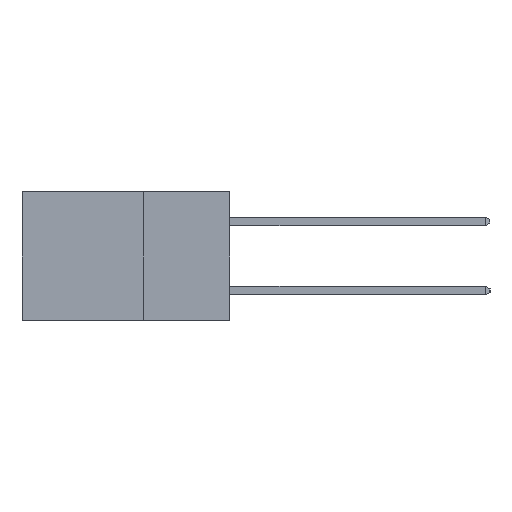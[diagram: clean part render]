
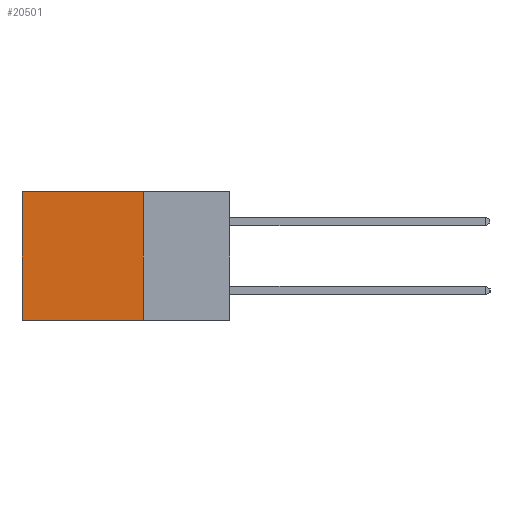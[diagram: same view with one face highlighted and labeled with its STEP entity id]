
A CAD part, left-side view. The second image highlights one B-rep face of the part: STEP entity #20501.
In plain terms, the highlighted planar face has unit normal (-1, 0, 0).
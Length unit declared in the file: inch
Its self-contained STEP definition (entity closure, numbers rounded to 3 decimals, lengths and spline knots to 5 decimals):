
#263 = CARTESIAN_POINT ( 'NONE',  ( 0.2615, 0.25, -0.37 ) ) ;
#494 = EDGE_CURVE ( 'NONE', #7256, #14960, #4353, .T. ) ;
#1299 = VERTEX_POINT ( 'NONE', #11297 ) ;
#1305 = CARTESIAN_POINT ( 'NONE',  ( 0.2615, 0.25, -0.37 ) ) ;
#1597 = FACE_OUTER_BOUND ( 'NONE', #7413, .T. ) ;
#2206 = LINE ( 'NONE', #10711, #11659 ) ;
#2581 = CARTESIAN_POINT ( 'NONE',  ( 0.2615, 0.25, -0.37 ) ) ;
#4353 = LINE ( 'NONE', #13115, #24732 ) ;
#5641 = EDGE_CURVE ( 'NONE', #7256, #10515, #22457, .T. ) ;
#6555 = DIRECTION ( 'NONE',  ( 1., 0., 0. ) ) ;
#7256 = VERTEX_POINT ( 'NONE', #17241 ) ;
#7413 = EDGE_LOOP ( 'NONE', ( #18184, #19885, #15107, #17958 ) ) ;
#7924 = VECTOR ( 'NONE', #14246, 39.37008 ) ;
#10231 = VECTOR ( 'NONE', #24812, 39.37008 ) ;
#10515 = VERTEX_POINT ( 'NONE', #10915 ) ;
#10711 = CARTESIAN_POINT ( 'NONE',  ( 0.2615, 0.6, -0.37 ) ) ;
#10915 = CARTESIAN_POINT ( 'NONE',  ( 0.2615, 0.25, -0.37 ) ) ;
#11297 = CARTESIAN_POINT ( 'NONE',  ( 0.2615, 0.6, -0.37 ) ) ;
#11659 = VECTOR ( 'NONE', #24363, 39.37008 ) ;
#13115 = CARTESIAN_POINT ( 'NONE',  ( 0.2615, 0.25, 0. ) ) ;
#14110 = EDGE_CURVE ( 'NONE', #14960, #1299, #2206, .T. ) ;
#14246 = DIRECTION ( 'NONE',  ( 0., 0., -1. ) ) ;
#14960 = VERTEX_POINT ( 'NONE', #22889 ) ;
#15107 = ORIENTED_EDGE ( 'NONE', *, *, #5641, .F. ) ;
#15469 = AXIS2_PLACEMENT_3D ( 'NONE', #2581, #6555, #20444 ) ;
#16150 = EDGE_CURVE ( 'NONE', #10515, #1299, #18854, .T. ) ;
#17241 = CARTESIAN_POINT ( 'NONE',  ( 0.2615, 0.25, 0. ) ) ;
#17958 = ORIENTED_EDGE ( 'NONE', *, *, #494, .T. ) ;
#18184 = ORIENTED_EDGE ( 'NONE', *, *, #14110, .T. ) ;
#18511 = PLANE ( 'NONE',  #15469 ) ;
#18854 = LINE ( 'NONE', #1305, #10231 ) ;
#19885 = ORIENTED_EDGE ( 'NONE', *, *, #16150, .F. ) ;
#20444 = DIRECTION ( 'NONE',  ( 0., 0., -1. ) ) ;
#20501 = ADVANCED_FACE ( 'NONE', ( #1597 ), #18511, .F. ) ;
#22457 = LINE ( 'NONE', #263, #7924 ) ;
#22889 = CARTESIAN_POINT ( 'NONE',  ( 0.2615, 0.6, 0. ) ) ;
#24363 = DIRECTION ( 'NONE',  ( 0., 0., -1. ) ) ;
#24732 = VECTOR ( 'NONE', #25443, 39.37008 ) ;
#24812 = DIRECTION ( 'NONE',  ( 0., 1., 0. ) ) ;
#25443 = DIRECTION ( 'NONE',  ( 0., 1., 0. ) ) ;
